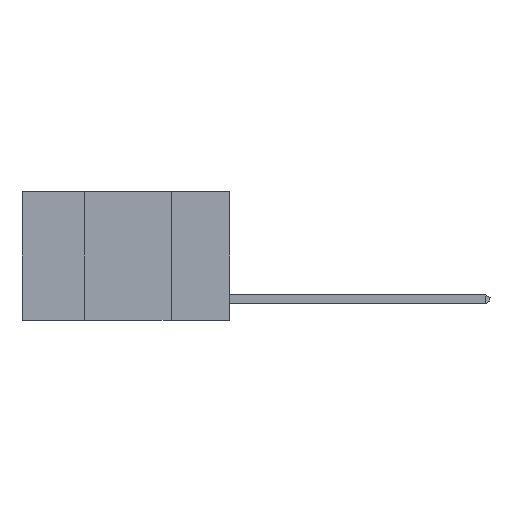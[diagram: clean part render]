
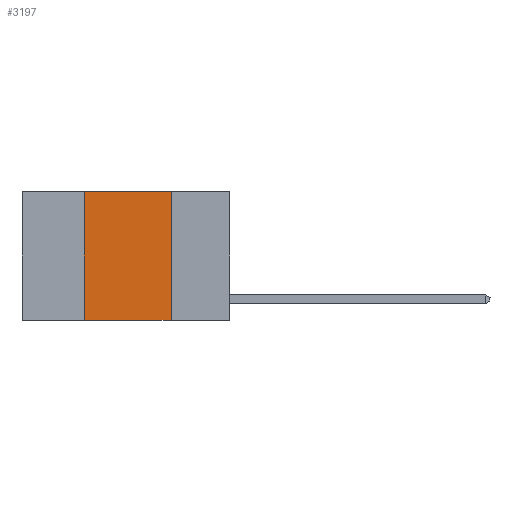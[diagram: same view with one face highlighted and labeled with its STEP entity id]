
A CAD part, left-side view. The second image highlights one B-rep face of the part: STEP entity #3197.
In plain terms, the highlighted planar face has unit normal (-1, 0, 0).
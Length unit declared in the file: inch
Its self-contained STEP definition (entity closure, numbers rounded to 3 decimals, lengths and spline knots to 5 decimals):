
#79 = VECTOR ( 'NONE', #4298, 39.37008 ) ;
#482 = AXIS2_PLACEMENT_3D ( 'NONE', #23636, #13558, #13797 ) ;
#524 = PLANE ( 'NONE',  #482 ) ;
#1763 = ORIENTED_EDGE ( 'NONE', *, *, #10126, .F. ) ;
#1771 = VERTEX_POINT ( 'NONE', #17248 ) ;
#3197 = ADVANCED_FACE ( 'NONE', ( #16004 ), #524, .F. ) ;
#3360 = LINE ( 'NONE', #10745, #18213 ) ;
#3541 = ORIENTED_EDGE ( 'NONE', *, *, #6272, .F. ) ;
#3853 = CARTESIAN_POINT ( 'NONE',  ( 0., 0.42, 0. ) ) ;
#4298 = DIRECTION ( 'NONE',  ( 0., -1., 0. ) ) ;
#4886 = DIRECTION ( 'NONE',  ( 0., -1., 0. ) ) ;
#5781 = VECTOR ( 'NONE', #15074, 39.37008 ) ;
#6168 = LINE ( 'NONE', #13774, #79 ) ;
#6272 = EDGE_CURVE ( 'NONE', #20327, #1771, #7489, .T. ) ;
#6866 = EDGE_CURVE ( 'NONE', #23465, #6932, #17655, .T. ) ;
#6932 = VERTEX_POINT ( 'NONE', #14153 ) ;
#7467 = ORIENTED_EDGE ( 'NONE', *, *, #18095, .T. ) ;
#7489 = LINE ( 'NONE', #3853, #5781 ) ;
#10126 = EDGE_CURVE ( 'NONE', #1771, #23465, #3360, .T. ) ;
#10745 = CARTESIAN_POINT ( 'NONE',  ( 0., 0.6, 0. ) ) ;
#11693 = DIRECTION ( 'NONE',  ( 0., 0., -1. ) ) ;
#12547 = VECTOR ( 'NONE', #11693, 39.37008 ) ;
#13558 = DIRECTION ( 'NONE',  ( 1., 0., 0. ) ) ;
#13774 = CARTESIAN_POINT ( 'NONE',  ( 0., 0.6, -0.37 ) ) ;
#13797 = DIRECTION ( 'NONE',  ( 0., 0., -1. ) ) ;
#14153 = CARTESIAN_POINT ( 'NONE',  ( 0., 0.17, -0.37 ) ) ;
#15074 = DIRECTION ( 'NONE',  ( 0., 0., 1. ) ) ;
#16004 = FACE_OUTER_BOUND ( 'NONE', #23334, .T. ) ;
#17248 = CARTESIAN_POINT ( 'NONE',  ( 0., 0.42, 0. ) ) ;
#17655 = LINE ( 'NONE', #23043, #12547 ) ;
#18095 = EDGE_CURVE ( 'NONE', #20327, #6932, #6168, .T. ) ;
#18213 = VECTOR ( 'NONE', #4886, 39.37008 ) ;
#20327 = VERTEX_POINT ( 'NONE', #23570 ) ;
#21103 = ORIENTED_EDGE ( 'NONE', *, *, #6866, .F. ) ;
#23043 = CARTESIAN_POINT ( 'NONE',  ( 0., 0.17, 0. ) ) ;
#23334 = EDGE_LOOP ( 'NONE', ( #21103, #1763, #3541, #7467 ) ) ;
#23465 = VERTEX_POINT ( 'NONE', #24386 ) ;
#23570 = CARTESIAN_POINT ( 'NONE',  ( 0., 0.42, -0.37 ) ) ;
#23636 = CARTESIAN_POINT ( 'NONE',  ( 0., 0.6, 0. ) ) ;
#24386 = CARTESIAN_POINT ( 'NONE',  ( 0., 0.17, 0. ) ) ;
